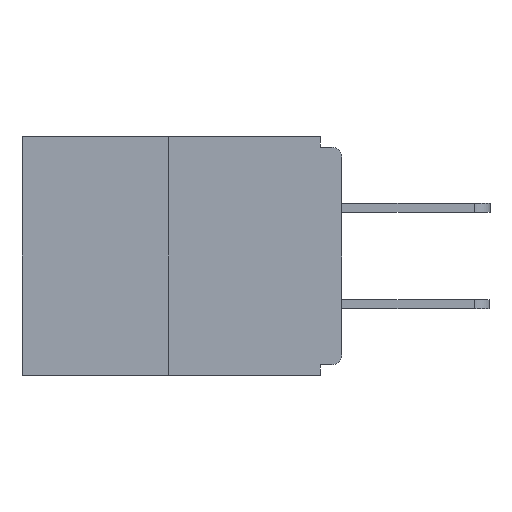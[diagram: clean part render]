
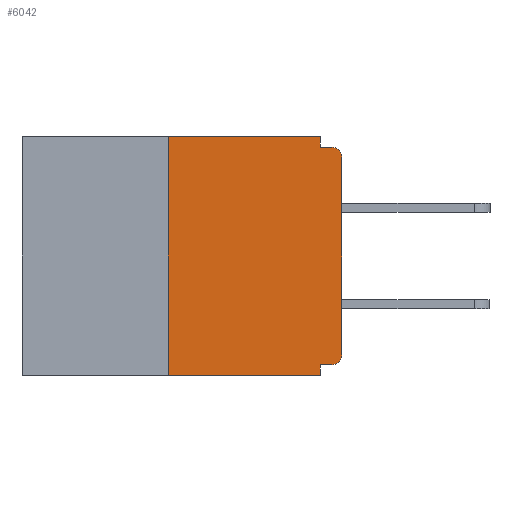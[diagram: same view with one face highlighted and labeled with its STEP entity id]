
A CAD part, left-side view. The second image highlights one B-rep face of the part: STEP entity #6042.
In plain terms, the highlighted planar face has unit normal (-1, 0, 0).
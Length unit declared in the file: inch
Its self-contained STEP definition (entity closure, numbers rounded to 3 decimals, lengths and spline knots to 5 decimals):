
#181 = VECTOR ( 'NONE', #3861, 39.37008 ) ;
#222 = CARTESIAN_POINT ( 'NONE',  ( 0., 0., -0.03 ) ) ;
#359 = EDGE_CURVE ( 'NONE', #745, #6159, #10011, .T. ) ;
#545 = DIRECTION ( 'NONE',  ( 0., 0., -1. ) ) ;
#745 = VERTEX_POINT ( 'NONE', #4680 ) ;
#937 = EDGE_CURVE ( 'NONE', #9546, #5085, #4910, .T. ) ;
#950 = DIRECTION ( 'NONE',  ( 0., 0., -1. ) ) ;
#1100 = CARTESIAN_POINT ( 'NONE',  ( 0., 0.46, -0.343 ) ) ;
#1204 = ORIENTED_EDGE ( 'NONE', *, *, #6516, .T. ) ;
#1284 = DIRECTION ( 'NONE',  ( -1., 0., 0. ) ) ;
#1340 = ORIENTED_EDGE ( 'NONE', *, *, #5041, .T. ) ;
#1359 = CARTESIAN_POINT ( 'NONE',  ( 0., 0.46, 0. ) ) ;
#1452 = LINE ( 'NONE', #6313, #181 ) ;
#1701 = EDGE_CURVE ( 'NONE', #5603, #8386, #3864, .T. ) ;
#1727 = ORIENTED_EDGE ( 'NONE', *, *, #8020, .F. ) ;
#1886 = DIRECTION ( 'NONE',  ( 0., 0., 1. ) ) ;
#1961 = ORIENTED_EDGE ( 'NONE', *, *, #359, .F. ) ;
#1965 = LINE ( 'NONE', #1359, #8928 ) ;
#2080 = VERTEX_POINT ( 'NONE', #222 ) ;
#2082 = CARTESIAN_POINT ( 'NONE',  ( 0., 0.015, -0.03 ) ) ;
#2130 = DIRECTION ( 'NONE',  ( 0., -1., 0. ) ) ;
#2183 = EDGE_LOOP ( 'NONE', ( #1727, #1961, #1204, #10689, #2340, #10194, #7328, #1340, #8252, #3372 ) ) ;
#2267 = VECTOR ( 'NONE', #8639, 39.37008 ) ;
#2333 = AXIS2_PLACEMENT_3D ( 'NONE', #8967, #3946, #545 ) ;
#2340 = ORIENTED_EDGE ( 'NONE', *, *, #1701, .F. ) ;
#2364 = DIRECTION ( 'NONE',  ( 1., 0., 0. ) ) ;
#2375 = VECTOR ( 'NONE', #6976, 39.37008 ) ;
#2564 = EDGE_CURVE ( 'NONE', #8908, #9546, #5129, .T. ) ;
#2753 = CARTESIAN_POINT ( 'NONE',  ( 0., 0.031, -0.015 ) ) ;
#2958 = VECTOR ( 'NONE', #4759, 39.37008 ) ;
#3014 = EDGE_CURVE ( 'NONE', #8386, #5442, #7886, .T. ) ;
#3214 = DIRECTION ( 'NONE',  ( 0., 0., -1. ) ) ;
#3338 = EDGE_CURVE ( 'NONE', #5603, #6801, #7253, .T. ) ;
#3372 = ORIENTED_EDGE ( 'NONE', *, *, #2564, .F. ) ;
#3454 = CARTESIAN_POINT ( 'NONE',  ( 0., 0.015, -0.328 ) ) ;
#3543 = CARTESIAN_POINT ( 'NONE',  ( 0., 0.25, 0. ) ) ;
#3559 = CARTESIAN_POINT ( 'NONE',  ( 0., 0.031, -0.343 ) ) ;
#3861 = DIRECTION ( 'NONE',  ( 0., 0., 1. ) ) ;
#3864 = LINE ( 'NONE', #9400, #2267 ) ;
#3946 = DIRECTION ( 'NONE',  ( -1., 0., 0. ) ) ;
#4395 = VECTOR ( 'NONE', #1886, 39.37008 ) ;
#4641 = DIRECTION ( 'NONE',  ( 0., 0., -1. ) ) ;
#4680 = CARTESIAN_POINT ( 'NONE',  ( 0., 0.25, -0.343 ) ) ;
#4759 = DIRECTION ( 'NONE',  ( 0., -1., 0. ) ) ;
#4829 = CARTESIAN_POINT ( 'NONE',  ( 0., 0.015, -0.015 ) ) ;
#4865 = CARTESIAN_POINT ( 'NONE',  ( 0., 0., -0.015 ) ) ;
#4910 = LINE ( 'NONE', #4865, #2958 ) ;
#5041 = EDGE_CURVE ( 'NONE', #2080, #5085, #8587, .T. ) ;
#5085 = VERTEX_POINT ( 'NONE', #4829 ) ;
#5129 = LINE ( 'NONE', #9297, #10338 ) ;
#5403 = LINE ( 'NONE', #1100, #2375 ) ;
#5442 = VERTEX_POINT ( 'NONE', #3559 ) ;
#5603 = VERTEX_POINT ( 'NONE', #3454 ) ;
#5937 = FACE_OUTER_BOUND ( 'NONE', #2183, .T. ) ;
#6042 = ADVANCED_FACE ( 'NONE', ( #5937 ), #8206, .F. ) ;
#6159 = VERTEX_POINT ( 'NONE', #10007 ) ;
#6313 = CARTESIAN_POINT ( 'NONE',  ( 0., 0., 0. ) ) ;
#6516 = EDGE_CURVE ( 'NONE', #745, #5442, #5403, .T. ) ;
#6801 = VERTEX_POINT ( 'NONE', #10751 ) ;
#6930 = DIRECTION ( 'NONE',  ( 0., 0., -1. ) ) ;
#6976 = DIRECTION ( 'NONE',  ( 0., -1., 0. ) ) ;
#7031 = EDGE_CURVE ( 'NONE', #6801, #2080, #1452, .T. ) ;
#7253 = CIRCLE ( 'NONE', #2333, 0.015 ) ;
#7260 = VECTOR ( 'NONE', #6930, 39.37008 ) ;
#7328 = ORIENTED_EDGE ( 'NONE', *, *, #7031, .T. ) ;
#7543 = CARTESIAN_POINT ( 'NONE',  ( 0., 0.031, -0.328 ) ) ;
#7886 = LINE ( 'NONE', #9394, #7260 ) ;
#8020 = EDGE_CURVE ( 'NONE', #6159, #8908, #1965, .T. ) ;
#8206 = PLANE ( 'NONE',  #10256 ) ;
#8251 = CARTESIAN_POINT ( 'NONE',  ( 0., 0.46, 0. ) ) ;
#8252 = ORIENTED_EDGE ( 'NONE', *, *, #937, .F. ) ;
#8386 = VERTEX_POINT ( 'NONE', #7543 ) ;
#8587 = CIRCLE ( 'NONE', #10273, 0.015 ) ;
#8639 = DIRECTION ( 'NONE',  ( 0., 1., 0. ) ) ;
#8908 = VERTEX_POINT ( 'NONE', #9270 ) ;
#8928 = VECTOR ( 'NONE', #2130, 39.37008 ) ;
#8967 = CARTESIAN_POINT ( 'NONE',  ( 0., 0.015, -0.313 ) ) ;
#9270 = CARTESIAN_POINT ( 'NONE',  ( 0., 0.031, 0. ) ) ;
#9297 = CARTESIAN_POINT ( 'NONE',  ( 0., 0.031, 0. ) ) ;
#9394 = CARTESIAN_POINT ( 'NONE',  ( 0., 0.031, -0.343 ) ) ;
#9400 = CARTESIAN_POINT ( 'NONE',  ( 0., 0., -0.328 ) ) ;
#9546 = VERTEX_POINT ( 'NONE', #2753 ) ;
#10007 = CARTESIAN_POINT ( 'NONE',  ( 0., 0.25, 0. ) ) ;
#10011 = LINE ( 'NONE', #3543, #4395 ) ;
#10194 = ORIENTED_EDGE ( 'NONE', *, *, #3338, .T. ) ;
#10256 = AXIS2_PLACEMENT_3D ( 'NONE', #8251, #2364, #3214 ) ;
#10273 = AXIS2_PLACEMENT_3D ( 'NONE', #2082, #1284, #4641 ) ;
#10338 = VECTOR ( 'NONE', #950, 39.37008 ) ;
#10689 = ORIENTED_EDGE ( 'NONE', *, *, #3014, .F. ) ;
#10751 = CARTESIAN_POINT ( 'NONE',  ( 0., 0., -0.313 ) ) ;
